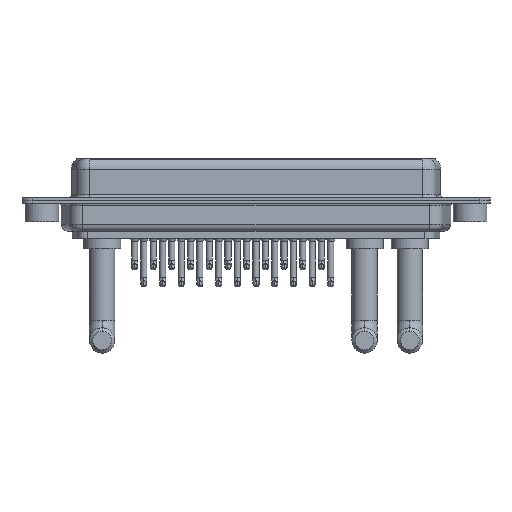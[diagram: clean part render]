
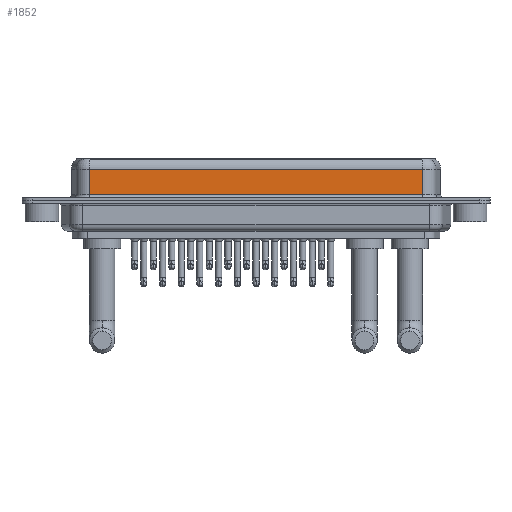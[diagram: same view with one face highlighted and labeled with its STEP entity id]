
A CAD part, front view. The second image highlights one B-rep face of the part: STEP entity #1852.
In plain terms, the highlighted planar face has unit normal (0, -1, 0).
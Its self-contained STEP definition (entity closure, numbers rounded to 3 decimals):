
#423 = VECTOR ( 'NONE', #15246, 1000. ) ;
#549 = VERTEX_POINT ( 'NONE', #16892 ) ;
#1222 = LINE ( 'NONE', #15713, #13199 ) ;
#1852 = ADVANCED_FACE ( 'NONE', ( #4458 ), #22593, .F. ) ;
#2129 = ORIENTED_EDGE ( 'NONE', *, *, #8118, .T. ) ;
#2997 = CARTESIAN_POINT ( 'NONE',  ( 56.462, -3.95, 4.65 ) ) ;
#3884 = LINE ( 'NONE', #5802, #423 ) ;
#3993 = VECTOR ( 'NONE', #9404, 1000. ) ;
#4458 = FACE_OUTER_BOUND ( 'NONE', #10765, .T. ) ;
#4975 = CARTESIAN_POINT ( 'NONE',  ( 7.038, -3.95, 6.4 ) ) ;
#5802 = CARTESIAN_POINT ( 'NONE',  ( 56.462, -3.95, 4.65 ) ) ;
#5891 = VERTEX_POINT ( 'NONE', #20139 ) ;
#6925 = LINE ( 'NONE', #14301, #16278 ) ;
#8118 = EDGE_CURVE ( 'NONE', #19009, #20499, #3884, .T. ) ;
#8195 = DIRECTION ( 'NONE',  ( 0., 0., 1. ) ) ;
#9404 = DIRECTION ( 'NONE',  ( 0., 0., -1. ) ) ;
#9682 = ORIENTED_EDGE ( 'NONE', *, *, #11968, .T. ) ;
#10141 = DIRECTION ( 'NONE',  ( 0., 0., -1. ) ) ;
#10653 = EDGE_CURVE ( 'NONE', #549, #5891, #6925, .T. ) ;
#10765 = EDGE_LOOP ( 'NONE', ( #23092, #2129, #9682, #21884 ) ) ;
#11968 = EDGE_CURVE ( 'NONE', #20499, #549, #18608, .T. ) ;
#13104 = CARTESIAN_POINT ( 'NONE',  ( 7.038, -3.95, 4.65 ) ) ;
#13199 = VECTOR ( 'NONE', #10141, 1000. ) ;
#14301 = CARTESIAN_POINT ( 'NONE',  ( 56.462, -3.95, 0.9 ) ) ;
#15246 = DIRECTION ( 'NONE',  ( -1., 0., 0. ) ) ;
#15449 = DIRECTION ( 'NONE',  ( 0., 1., 0. ) ) ;
#15713 = CARTESIAN_POINT ( 'NONE',  ( 56.462, -3.95, 6.4 ) ) ;
#16278 = VECTOR ( 'NONE', #17707, 1000. ) ;
#16892 = CARTESIAN_POINT ( 'NONE',  ( 7.038, -3.95, 0.9 ) ) ;
#17707 = DIRECTION ( 'NONE',  ( 1., 0., 0. ) ) ;
#18608 = LINE ( 'NONE', #4975, #3993 ) ;
#19009 = VERTEX_POINT ( 'NONE', #2997 ) ;
#19092 = CARTESIAN_POINT ( 'NONE',  ( 56.462, -3.95, 6.4 ) ) ;
#20139 = CARTESIAN_POINT ( 'NONE',  ( 56.462, -3.95, 0.9 ) ) ;
#20499 = VERTEX_POINT ( 'NONE', #13104 ) ;
#21731 = EDGE_CURVE ( 'NONE', #19009, #5891, #1222, .T. ) ;
#21884 = ORIENTED_EDGE ( 'NONE', *, *, #10653, .T. ) ;
#22593 = PLANE ( 'NONE',  #22921 ) ;
#22921 = AXIS2_PLACEMENT_3D ( 'NONE', #19092, #15449, #8195 ) ;
#23092 = ORIENTED_EDGE ( 'NONE', *, *, #21731, .F. ) ;
